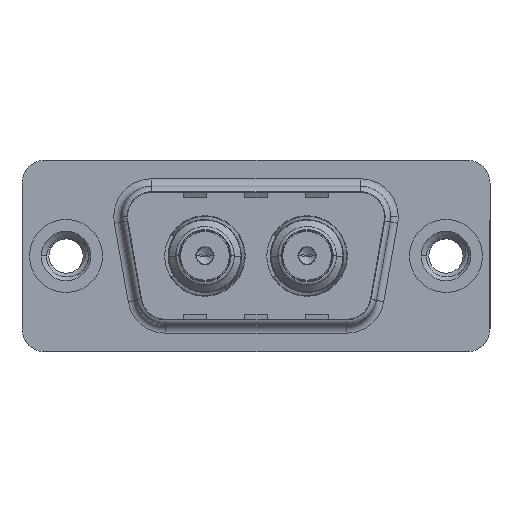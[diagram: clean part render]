
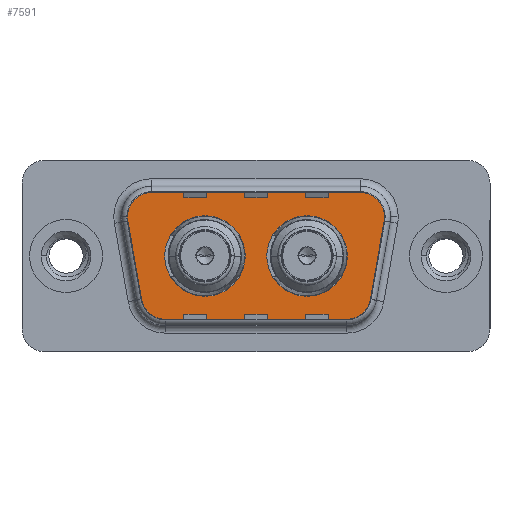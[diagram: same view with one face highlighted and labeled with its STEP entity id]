
A CAD part, top view. The second image highlights one B-rep face of the part: STEP entity #7591.
In plain terms, the highlighted planar face has unit normal (0, 0, 1).
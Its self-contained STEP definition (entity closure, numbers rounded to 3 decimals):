
#105 = ORIENTED_EDGE ( 'NONE', *, *, #7107, .F. ) ;
#138 = EDGE_CURVE ( 'NONE', #12380, #12208, #2108, .T. ) ;
#156 = CARTESIAN_POINT ( 'NONE',  ( 3.466, 2.553, 0. ) ) ;
#158 = VERTEX_POINT ( 'NONE', #156 ) ;
#235 = CARTESIAN_POINT ( 'NONE',  ( 4.489, -3.247, 0. ) ) ;
#466 = ORIENTED_EDGE ( 'NONE', *, *, #8399, .T. ) ;
#533 = DIRECTION ( 'NONE',  ( 0., 0., 1. ) ) ;
#658 = ORIENTED_EDGE ( 'NONE', *, *, #138, .T. ) ;
#885 = ORIENTED_EDGE ( 'NONE', *, *, #11137, .T. ) ;
#930 = CARTESIAN_POINT ( 'NONE',  ( 15.86, 0., 0. ) ) ;
#1048 = EDGE_LOOP ( 'NONE', ( #12477, #6107 ) ) ;
#1126 = CARTESIAN_POINT ( 'NONE',  ( 18.541, -4.9, 0. ) ) ;
#1388 = DIRECTION ( 'NONE',  ( 0.174, -0.985, 0. ) ) ;
#1498 = EDGE_CURVE ( 'NONE', #14141, #8274, #10510, .T. ) ;
#1966 = CARTESIAN_POINT ( 'NONE',  ( 15.86, 0., 0. ) ) ;
#2102 = DIRECTION ( 'NONE',  ( 1., 0., 0. ) ) ;
#2108 = LINE ( 'NONE', #10663, #13752 ) ;
#2122 = ORIENTED_EDGE ( 'NONE', *, *, #6860, .T. ) ;
#2161 = VERTEX_POINT ( 'NONE', #5007 ) ;
#2202 = PLANE ( 'NONE',  #13135 ) ;
#2713 = DIRECTION ( 'NONE',  ( 0., 0., 1. ) ) ;
#2793 = AXIS2_PLACEMENT_3D ( 'NONE', #1966, #9979, #3115 ) ;
#2906 = VERTEX_POINT ( 'NONE', #10997 ) ;
#3115 = DIRECTION ( 'NONE',  ( 1., 0., 0. ) ) ;
#3156 = CIRCLE ( 'NONE', #5257, 2. ) ;
#3206 = EDGE_CURVE ( 'NONE', #2906, #2161, #3156, .T. ) ;
#3209 = VECTOR ( 'NONE', #1388, 1000. ) ;
#3220 = EDGE_LOOP ( 'NONE', ( #105, #9604 ) ) ;
#3473 = DIRECTION ( 'NONE',  ( -1., 0., 0. ) ) ;
#3516 = EDGE_CURVE ( 'NONE', #11916, #10016, #9427, .T. ) ;
#3529 = VECTOR ( 'NONE', #14657, 1000. ) ;
#3696 = FACE_BOUND ( 'NONE', #3220, .T. ) ;
#3705 = CARTESIAN_POINT ( 'NONE',  ( 3.466, 2.553, 0. ) ) ;
#3946 = CARTESIAN_POINT ( 'NONE',  ( 19.564, 2.9, 0. ) ) ;
#4069 = CIRCLE ( 'NONE', #14448, 2.65 ) ;
#4171 = DIRECTION ( 'NONE',  ( 1., 0., 0. ) ) ;
#4410 = AXIS2_PLACEMENT_3D ( 'NONE', #3946, #533, #3473 ) ;
#4513 = CARTESIAN_POINT ( 'NONE',  ( 18.541, -2.9, 0. ) ) ;
#4839 = CARTESIAN_POINT ( 'NONE',  ( 9.14, 0., 0. ) ) ;
#4939 = VECTOR ( 'NONE', #11844, 1000. ) ;
#5007 = CARTESIAN_POINT ( 'NONE',  ( 19.564, 4.9, 0. ) ) ;
#5215 = ORIENTED_EDGE ( 'NONE', *, *, #5296, .T. ) ;
#5257 = AXIS2_PLACEMENT_3D ( 'NONE', #13559, #6828, #14121 ) ;
#5296 = EDGE_CURVE ( 'NONE', #14376, #12858, #6513, .T. ) ;
#5381 = CARTESIAN_POINT ( 'NONE',  ( 21.534, 2.553, 0. ) ) ;
#5452 = EDGE_CURVE ( 'NONE', #12208, #2906, #13814, .T. ) ;
#5553 = CARTESIAN_POINT ( 'NONE',  ( 6.49, 0., 0. ) ) ;
#5999 = DIRECTION ( 'NONE',  ( 1., 0., 0. ) ) ;
#6107 = ORIENTED_EDGE ( 'NONE', *, *, #12218, .F. ) ;
#6152 = CARTESIAN_POINT ( 'NONE',  ( 18.51, 0., 0. ) ) ;
#6212 = EDGE_CURVE ( 'NONE', #7548, #158, #8056, .T. ) ;
#6513 = CIRCLE ( 'NONE', #9333, 2. ) ;
#6828 = DIRECTION ( 'NONE',  ( 0., 0., 1. ) ) ;
#6842 = DIRECTION ( 'NONE',  ( 1., 0., 0. ) ) ;
#6860 = EDGE_CURVE ( 'NONE', #12858, #12469, #9989, .T. ) ;
#7107 = EDGE_CURVE ( 'NONE', #8274, #14141, #4069, .T. ) ;
#7390 = DIRECTION ( 'NONE',  ( 0.174, 0.985, 0. ) ) ;
#7548 = VERTEX_POINT ( 'NONE', #7840 ) ;
#7591 = ADVANCED_FACE ( 'NONE', ( #9787, #3696, #13510 ), #2202, .T. ) ;
#7801 = DIRECTION ( 'NONE',  ( 0., 0., 1. ) ) ;
#7840 = CARTESIAN_POINT ( 'NONE',  ( 5.436, 4.9, 0. ) ) ;
#7880 = ORIENTED_EDGE ( 'NONE', *, *, #5452, .T. ) ;
#7910 = ORIENTED_EDGE ( 'NONE', *, *, #6212, .T. ) ;
#8056 = CIRCLE ( 'NONE', #13799, 2. ) ;
#8075 = AXIS2_PLACEMENT_3D ( 'NONE', #930, #10115, #2102 ) ;
#8239 = CARTESIAN_POINT ( 'NONE',  ( 11.79, 0., 0. ) ) ;
#8274 = VERTEX_POINT ( 'NONE', #8239 ) ;
#8399 = EDGE_CURVE ( 'NONE', #2161, #7548, #14034, .T. ) ;
#8837 = CARTESIAN_POINT ( 'NONE',  ( 6.459, -2.9, 0. ) ) ;
#8878 = CARTESIAN_POINT ( 'NONE',  ( 6.459, -4.9, 0. ) ) ;
#9328 = AXIS2_PLACEMENT_3D ( 'NONE', #9556, #2713, #10699 ) ;
#9333 = AXIS2_PLACEMENT_3D ( 'NONE', #8837, #14122, #14197 ) ;
#9412 = DIRECTION ( 'NONE',  ( 0., 0., 1. ) ) ;
#9427 = CIRCLE ( 'NONE', #8075, 2.65 ) ;
#9463 = CARTESIAN_POINT ( 'NONE',  ( 9.14, 0., 0. ) ) ;
#9483 = ORIENTED_EDGE ( 'NONE', *, *, #14770, .T. ) ;
#9556 = CARTESIAN_POINT ( 'NONE',  ( 18.541, -2.9, 0. ) ) ;
#9604 = ORIENTED_EDGE ( 'NONE', *, *, #1498, .F. ) ;
#9747 = AXIS2_PLACEMENT_3D ( 'NONE', #9463, #9412, #11081 ) ;
#9787 = FACE_BOUND ( 'NONE', #1048, .T. ) ;
#9979 = DIRECTION ( 'NONE',  ( 0., 0., 1. ) ) ;
#9989 = LINE ( 'NONE', #13502, #3529 ) ;
#10016 = VERTEX_POINT ( 'NONE', #11602 ) ;
#10115 = DIRECTION ( 'NONE',  ( 0., 0., 1. ) ) ;
#10224 = ORIENTED_EDGE ( 'NONE', *, *, #3206, .T. ) ;
#10510 = CIRCLE ( 'NONE', #9747, 2.65 ) ;
#10663 = CARTESIAN_POINT ( 'NONE',  ( 21.534, 2.553, 0. ) ) ;
#10699 = DIRECTION ( 'NONE',  ( 1., 0., 0. ) ) ;
#10717 = CARTESIAN_POINT ( 'NONE',  ( 5.436, 4.9, 0. ) ) ;
#10997 = CARTESIAN_POINT ( 'NONE',  ( 21.564, 2.9, 0. ) ) ;
#11081 = DIRECTION ( 'NONE',  ( 1., 0., 0. ) ) ;
#11093 = EDGE_LOOP ( 'NONE', ( #885, #658, #7880, #10224, #466, #7910, #9483, #5215, #2122 ) ) ;
#11137 = EDGE_CURVE ( 'NONE', #12469, #12380, #13491, .T. ) ;
#11511 = CIRCLE ( 'NONE', #2793, 2.65 ) ;
#11602 = CARTESIAN_POINT ( 'NONE',  ( 13.21, 0., 0. ) ) ;
#11609 = LINE ( 'NONE', #3705, #3209 ) ;
#11663 = CARTESIAN_POINT ( 'NONE',  ( 5.436, 2.9, 0. ) ) ;
#11844 = DIRECTION ( 'NONE',  ( -1., 0., 0. ) ) ;
#11916 = VERTEX_POINT ( 'NONE', #6152 ) ;
#12208 = VERTEX_POINT ( 'NONE', #5381 ) ;
#12218 = EDGE_CURVE ( 'NONE', #10016, #11916, #11511, .T. ) ;
#12380 = VERTEX_POINT ( 'NONE', #14680 ) ;
#12469 = VERTEX_POINT ( 'NONE', #1126 ) ;
#12477 = ORIENTED_EDGE ( 'NONE', *, *, #3516, .F. ) ;
#12805 = DIRECTION ( 'NONE',  ( 0., 0., 1. ) ) ;
#12858 = VERTEX_POINT ( 'NONE', #8878 ) ;
#13135 = AXIS2_PLACEMENT_3D ( 'NONE', #4513, #13631, #6842 ) ;
#13491 = CIRCLE ( 'NONE', #9328, 2. ) ;
#13502 = CARTESIAN_POINT ( 'NONE',  ( 6.459, -4.9, 0. ) ) ;
#13510 = FACE_OUTER_BOUND ( 'NONE', #11093, .T. ) ;
#13559 = CARTESIAN_POINT ( 'NONE',  ( 19.564, 2.9, 0. ) ) ;
#13631 = DIRECTION ( 'NONE',  ( 0., 0., 1. ) ) ;
#13752 = VECTOR ( 'NONE', #7390, 1000. ) ;
#13799 = AXIS2_PLACEMENT_3D ( 'NONE', #11663, #7801, #4171 ) ;
#13814 = CIRCLE ( 'NONE', #4410, 2. ) ;
#14034 = LINE ( 'NONE', #10717, #4939 ) ;
#14121 = DIRECTION ( 'NONE',  ( -1., 0., 0. ) ) ;
#14122 = DIRECTION ( 'NONE',  ( 0., 0., 1. ) ) ;
#14141 = VERTEX_POINT ( 'NONE', #5553 ) ;
#14197 = DIRECTION ( 'NONE',  ( -1., 0., 0. ) ) ;
#14376 = VERTEX_POINT ( 'NONE', #235 ) ;
#14448 = AXIS2_PLACEMENT_3D ( 'NONE', #4839, #12805, #5999 ) ;
#14657 = DIRECTION ( 'NONE',  ( 1., 0., 0. ) ) ;
#14680 = CARTESIAN_POINT ( 'NONE',  ( 20.511, -3.247, 0. ) ) ;
#14770 = EDGE_CURVE ( 'NONE', #158, #14376, #11609, .T. ) ;
